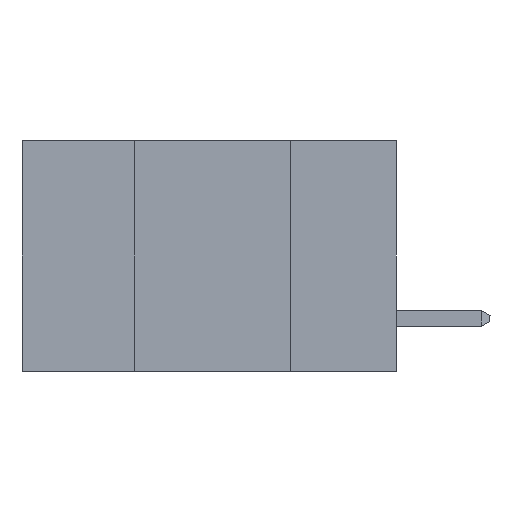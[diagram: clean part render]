
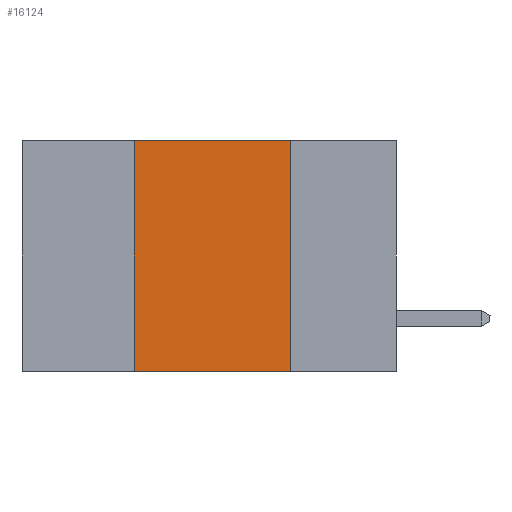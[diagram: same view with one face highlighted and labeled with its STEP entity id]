
A CAD part, left-side view. The second image highlights one B-rep face of the part: STEP entity #16124.
In plain terms, the highlighted planar face has unit normal (-1, 0, 0).
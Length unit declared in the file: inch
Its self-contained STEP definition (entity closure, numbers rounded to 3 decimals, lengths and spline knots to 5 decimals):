
#122 = AXIS2_PLACEMENT_3D ( 'NONE', #226, #13770, #4728 ) ;
#151 = ORIENTED_EDGE ( 'NONE', *, *, #8677, .F. ) ;
#226 = CARTESIAN_POINT ( 'NONE',  ( 0., 0.6, 0. ) ) ;
#1985 = EDGE_CURVE ( 'NONE', #4953, #12231, #18757, .T. ) ;
#2953 = CARTESIAN_POINT ( 'NONE',  ( 0., 0.42, 0. ) ) ;
#2991 = EDGE_CURVE ( 'NONE', #4953, #19090, #13387, .T. ) ;
#3431 = VECTOR ( 'NONE', #8925, 39.37008 ) ;
#3852 = VECTOR ( 'NONE', #17455, 39.37008 ) ;
#4079 = CARTESIAN_POINT ( 'NONE',  ( 0., 0.17, -0.37 ) ) ;
#4728 = DIRECTION ( 'NONE',  ( 0., 0., -1. ) ) ;
#4953 = VERTEX_POINT ( 'NONE', #13037 ) ;
#5508 = ORIENTED_EDGE ( 'NONE', *, *, #1985, .T. ) ;
#7005 = VERTEX_POINT ( 'NONE', #7340 ) ;
#7340 = CARTESIAN_POINT ( 'NONE',  ( 0., 0.17, 0. ) ) ;
#8677 = EDGE_CURVE ( 'NONE', #19090, #7005, #19049, .T. ) ;
#8925 = DIRECTION ( 'NONE',  ( 0., -1., 0. ) ) ;
#9059 = CARTESIAN_POINT ( 'NONE',  ( 0., 0.6, 0. ) ) ;
#10694 = PLANE ( 'NONE',  #122 ) ;
#12231 = VERTEX_POINT ( 'NONE', #13701 ) ;
#12593 = ORIENTED_EDGE ( 'NONE', *, *, #2991, .F. ) ;
#13037 = CARTESIAN_POINT ( 'NONE',  ( 0., 0.42, -0.37 ) ) ;
#13045 = FACE_OUTER_BOUND ( 'NONE', #13339, .T. ) ;
#13339 = EDGE_LOOP ( 'NONE', ( #15131, #151, #12593, #5508 ) ) ;
#13387 = LINE ( 'NONE', #14123, #17210 ) ;
#13701 = CARTESIAN_POINT ( 'NONE',  ( 0., 0.17, -0.37 ) ) ;
#13770 = DIRECTION ( 'NONE',  ( 1., 0., 0. ) ) ;
#14102 = DIRECTION ( 'NONE',  ( 0., 0., 1. ) ) ;
#14123 = CARTESIAN_POINT ( 'NONE',  ( 0., 0.42, -0.37 ) ) ;
#15131 = ORIENTED_EDGE ( 'NONE', *, *, #16342, .F. ) ;
#16124 = ADVANCED_FACE ( 'NONE', ( #13045 ), #10694, .F. ) ;
#16213 = LINE ( 'NONE', #4079, #3852 ) ;
#16342 = EDGE_CURVE ( 'NONE', #7005, #12231, #16213, .T. ) ;
#17210 = VECTOR ( 'NONE', #14102, 39.37008 ) ;
#17455 = DIRECTION ( 'NONE',  ( 0., 0., -1. ) ) ;
#17573 = CARTESIAN_POINT ( 'NONE',  ( 0., 0.6, -0.37 ) ) ;
#17859 = DIRECTION ( 'NONE',  ( 0., -1., 0. ) ) ;
#18346 = VECTOR ( 'NONE', #17859, 39.37008 ) ;
#18757 = LINE ( 'NONE', #17573, #18346 ) ;
#19049 = LINE ( 'NONE', #9059, #3431 ) ;
#19090 = VERTEX_POINT ( 'NONE', #2953 ) ;
